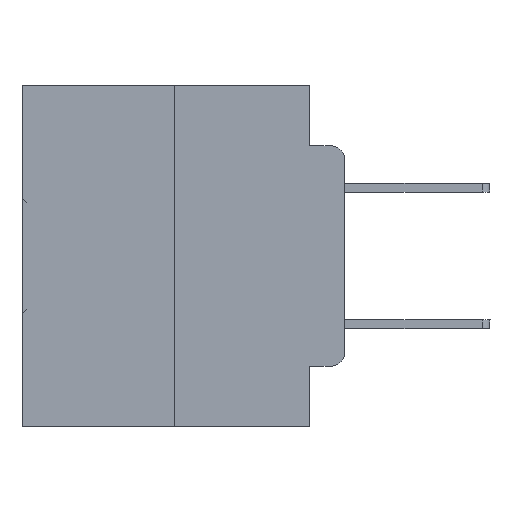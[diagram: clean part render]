
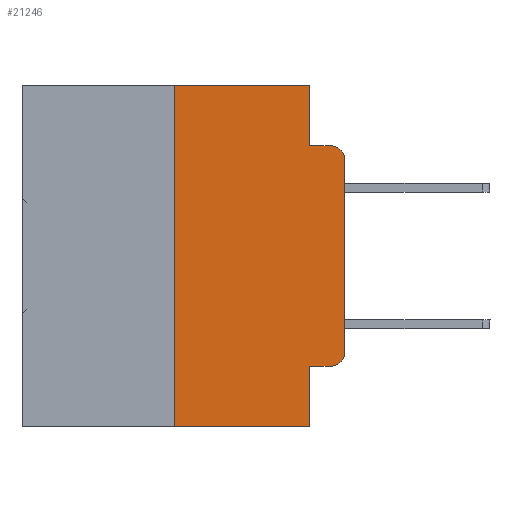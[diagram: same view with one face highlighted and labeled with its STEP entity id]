
A CAD part, left-side view. The second image highlights one B-rep face of the part: STEP entity #21246.
In plain terms, the highlighted planar face has unit normal (-1, 0, 0).
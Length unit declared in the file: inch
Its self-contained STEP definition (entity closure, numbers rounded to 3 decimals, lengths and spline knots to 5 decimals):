
#900 = VERTEX_POINT ( 'NONE', #4553 ) ;
#1309 = EDGE_CURVE ( 'NONE', #4163, #4111, #17081, .T. ) ;
#1674 = DIRECTION ( 'NONE',  ( 0., -1., 0. ) ) ;
#2224 = EDGE_CURVE ( 'NONE', #4111, #900, #18010, .T. ) ;
#2230 = FACE_OUTER_BOUND ( 'NONE', #9781, .T. ) ;
#2268 = CARTESIAN_POINT ( 'NONE',  ( 0., 0., -0.1085 ) ) ;
#3298 = EDGE_CURVE ( 'NONE', #9222, #13821, #7305, .T. ) ;
#3453 = CARTESIAN_POINT ( 'NONE',  ( 0., 0.25, 0. ) ) ;
#3459 = CARTESIAN_POINT ( 'NONE',  ( 0., 0.02, -0.0885 ) ) ;
#4111 = VERTEX_POINT ( 'NONE', #3453 ) ;
#4163 = VERTEX_POINT ( 'NONE', #9552 ) ;
#4553 = CARTESIAN_POINT ( 'NONE',  ( 0., 0.051, 0. ) ) ;
#4747 = DIRECTION ( 'NONE',  ( -1., 0., 0. ) ) ;
#5116 = CARTESIAN_POINT ( 'NONE',  ( 0., 0.473, 0. ) ) ;
#5552 = CARTESIAN_POINT ( 'NONE',  ( 0., 0.051, -0.0885 ) ) ;
#6496 = EDGE_CURVE ( 'NONE', #13821, #7669, #6693, .T. ) ;
#6693 = CIRCLE ( 'NONE', #19304, 0.02 ) ;
#6915 = EDGE_CURVE ( 'NONE', #25662, #10829, #21219, .T. ) ;
#6923 = VECTOR ( 'NONE', #23629, 39.37008 ) ;
#7094 = DIRECTION ( 'NONE',  ( 0., 0., -1. ) ) ;
#7232 = CARTESIAN_POINT ( 'NONE',  ( 0., 0., -0.3915 ) ) ;
#7305 = LINE ( 'NONE', #27044, #6923 ) ;
#7637 = ORIENTED_EDGE ( 'NONE', *, *, #2224, .F. ) ;
#7669 = VERTEX_POINT ( 'NONE', #3459 ) ;
#9222 = VERTEX_POINT ( 'NONE', #7232 ) ;
#9552 = CARTESIAN_POINT ( 'NONE',  ( 0., 0.25, -0.5 ) ) ;
#9781 = EDGE_LOOP ( 'NONE', ( #29775, #21678, #26902, #18042, #7637, #34355, #26844, #28564, #19069, #14877 ) ) ;
#10479 = CIRCLE ( 'NONE', #12761, 0.02 ) ;
#10829 = VERTEX_POINT ( 'NONE', #28926 ) ;
#11004 = DIRECTION ( 'NONE',  ( 0., -1., 0. ) ) ;
#11688 = DIRECTION ( 'NONE',  ( 0., 0., -1. ) ) ;
#12052 = CARTESIAN_POINT ( 'NONE',  ( 0., 0.051, 0. ) ) ;
#12236 = VECTOR ( 'NONE', #13308, 39.37008 ) ;
#12527 = DIRECTION ( 'NONE',  ( -1., 0., 0. ) ) ;
#12761 = AXIS2_PLACEMENT_3D ( 'NONE', #15520, #4747, #26120 ) ;
#12906 = EDGE_CURVE ( 'NONE', #25662, #16436, #24430, .T. ) ;
#13193 = PLANE ( 'NONE',  #14229 ) ;
#13308 = DIRECTION ( 'NONE',  ( 0., -1., 0. ) ) ;
#13821 = VERTEX_POINT ( 'NONE', #2268 ) ;
#14229 = AXIS2_PLACEMENT_3D ( 'NONE', #5116, #31675, #7094 ) ;
#14877 = ORIENTED_EDGE ( 'NONE', *, *, #29619, .T. ) ;
#15520 = CARTESIAN_POINT ( 'NONE',  ( 0., 0.02, -0.3915 ) ) ;
#15828 = VECTOR ( 'NONE', #11688, 39.37008 ) ;
#16436 = VERTEX_POINT ( 'NONE', #18094 ) ;
#17081 = LINE ( 'NONE', #28583, #29052 ) ;
#17398 = EDGE_CURVE ( 'NONE', #31699, #7669, #19017, .T. ) ;
#18010 = LINE ( 'NONE', #28981, #29874 ) ;
#18042 = ORIENTED_EDGE ( 'NONE', *, *, #35087, .F. ) ;
#18094 = CARTESIAN_POINT ( 'NONE',  ( 0., 0.02, -0.4115 ) ) ;
#19017 = LINE ( 'NONE', #5552, #23277 ) ;
#19039 = CARTESIAN_POINT ( 'NONE',  ( 0., 0.051, -0.4115 ) ) ;
#19069 = ORIENTED_EDGE ( 'NONE', *, *, #12906, .T. ) ;
#19304 = AXIS2_PLACEMENT_3D ( 'NONE', #26168, #12527, #23640 ) ;
#21219 = LINE ( 'NONE', #31989, #26211 ) ;
#21246 = ADVANCED_FACE ( 'NONE', ( #2230 ), #13193, .F. ) ;
#21678 = ORIENTED_EDGE ( 'NONE', *, *, #6496, .T. ) ;
#21879 = DIRECTION ( 'NONE',  ( 0., -1., 0. ) ) ;
#22113 = LINE ( 'NONE', #27179, #29948 ) ;
#23277 = VECTOR ( 'NONE', #21879, 39.37008 ) ;
#23629 = DIRECTION ( 'NONE',  ( 0., 0., 1. ) ) ;
#23640 = DIRECTION ( 'NONE',  ( 0., 0., -1. ) ) ;
#24430 = LINE ( 'NONE', #19039, #12236 ) ;
#25662 = VERTEX_POINT ( 'NONE', #26098 ) ;
#26098 = CARTESIAN_POINT ( 'NONE',  ( 0., 0.051, -0.4115 ) ) ;
#26120 = DIRECTION ( 'NONE',  ( 0., 0., -1. ) ) ;
#26168 = CARTESIAN_POINT ( 'NONE',  ( 0., 0.02, -0.1085 ) ) ;
#26211 = VECTOR ( 'NONE', #29309, 39.37008 ) ;
#26844 = ORIENTED_EDGE ( 'NONE', *, *, #29769, .T. ) ;
#26902 = ORIENTED_EDGE ( 'NONE', *, *, #17398, .F. ) ;
#26972 = CARTESIAN_POINT ( 'NONE',  ( 0., 0.051, -0.0885 ) ) ;
#27044 = CARTESIAN_POINT ( 'NONE',  ( 0., 0., 0. ) ) ;
#27179 = CARTESIAN_POINT ( 'NONE',  ( 0., 0.473, -0.5 ) ) ;
#28564 = ORIENTED_EDGE ( 'NONE', *, *, #6915, .F. ) ;
#28583 = CARTESIAN_POINT ( 'NONE',  ( 0., 0.25, 0. ) ) ;
#28753 = LINE ( 'NONE', #12052, #15828 ) ;
#28926 = CARTESIAN_POINT ( 'NONE',  ( 0., 0.051, -0.5 ) ) ;
#28981 = CARTESIAN_POINT ( 'NONE',  ( 0., 0.473, 0. ) ) ;
#29052 = VECTOR ( 'NONE', #31250, 39.37008 ) ;
#29309 = DIRECTION ( 'NONE',  ( 0., 0., -1. ) ) ;
#29619 = EDGE_CURVE ( 'NONE', #16436, #9222, #10479, .T. ) ;
#29769 = EDGE_CURVE ( 'NONE', #4163, #10829, #22113, .T. ) ;
#29775 = ORIENTED_EDGE ( 'NONE', *, *, #3298, .T. ) ;
#29874 = VECTOR ( 'NONE', #1674, 39.37008 ) ;
#29948 = VECTOR ( 'NONE', #11004, 39.37008 ) ;
#31250 = DIRECTION ( 'NONE',  ( 0., 0., 1. ) ) ;
#31675 = DIRECTION ( 'NONE',  ( 1., 0., 0. ) ) ;
#31699 = VERTEX_POINT ( 'NONE', #26972 ) ;
#31989 = CARTESIAN_POINT ( 'NONE',  ( 0., 0.051, 0. ) ) ;
#34355 = ORIENTED_EDGE ( 'NONE', *, *, #1309, .F. ) ;
#35087 = EDGE_CURVE ( 'NONE', #900, #31699, #28753, .T. ) ;
